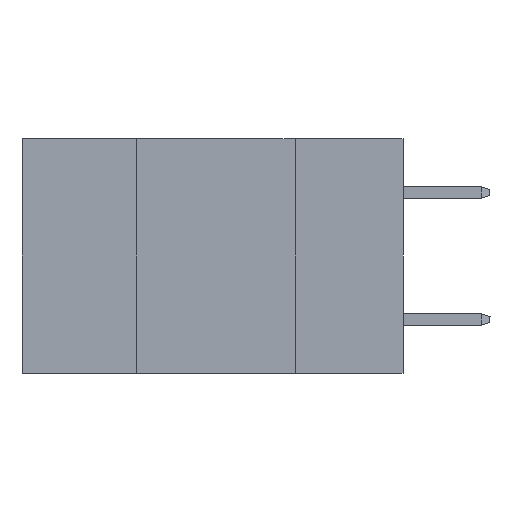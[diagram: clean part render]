
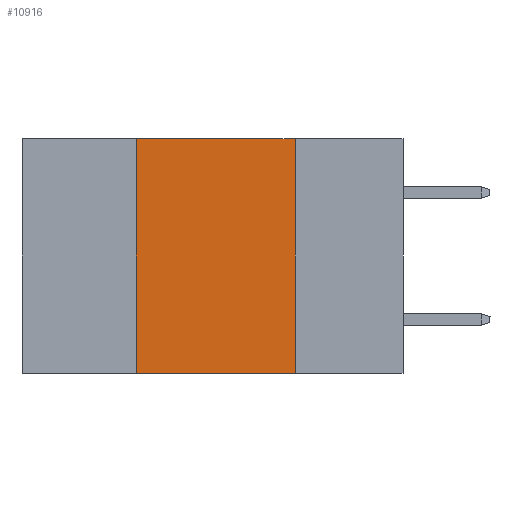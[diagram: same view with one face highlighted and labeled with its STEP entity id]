
A CAD part, left-side view. The second image highlights one B-rep face of the part: STEP entity #10916.
In plain terms, the highlighted planar face has unit normal (-1, 0, 0).
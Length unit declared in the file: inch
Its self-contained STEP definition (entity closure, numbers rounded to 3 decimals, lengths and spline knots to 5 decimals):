
#1675 = DIRECTION ( 'NONE',  ( 1., 0., 0. ) ) ;
#2633 = ORIENTED_EDGE ( 'NONE', *, *, #18885, .F. ) ;
#2917 = VECTOR ( 'NONE', #20141, 39.37008 ) ;
#5406 = LINE ( 'NONE', #11990, #14922 ) ;
#6867 = EDGE_CURVE ( 'NONE', #15799, #18424, #5406, .T. ) ;
#7306 = LINE ( 'NONE', #20338, #10211 ) ;
#7468 = EDGE_LOOP ( 'NONE', ( #17156, #2633, #8340, #9857 ) ) ;
#7472 = VECTOR ( 'NONE', #13784, 39.37008 ) ;
#7933 = FACE_OUTER_BOUND ( 'NONE', #7468, .T. ) ;
#8136 = VERTEX_POINT ( 'NONE', #20972 ) ;
#8340 = ORIENTED_EDGE ( 'NONE', *, *, #14727, .F. ) ;
#8934 = LINE ( 'NONE', #11950, #7472 ) ;
#9857 = ORIENTED_EDGE ( 'NONE', *, *, #11999, .T. ) ;
#9863 = PLANE ( 'NONE',  #14648 ) ;
#10211 = VECTOR ( 'NONE', #13676, 39.37008 ) ;
#10916 = ADVANCED_FACE ( 'NONE', ( #7933 ), #9863, .F. ) ;
#11162 = CARTESIAN_POINT ( 'NONE',  ( 0., 0.6, 0. ) ) ;
#11702 = CARTESIAN_POINT ( 'NONE',  ( 0., 0.17, -0.37 ) ) ;
#11835 = CARTESIAN_POINT ( 'NONE',  ( 0., 0.42, 0. ) ) ;
#11950 = CARTESIAN_POINT ( 'NONE',  ( 0., 0.42, 0. ) ) ;
#11990 = CARTESIAN_POINT ( 'NONE',  ( 0., 0.17, 0. ) ) ;
#11999 = EDGE_CURVE ( 'NONE', #8136, #18424, #7306, .T. ) ;
#13385 = LINE ( 'NONE', #18405, #2917 ) ;
#13676 = DIRECTION ( 'NONE',  ( 0., -1., 0. ) ) ;
#13784 = DIRECTION ( 'NONE',  ( 0., 0., 1. ) ) ;
#14450 = CARTESIAN_POINT ( 'NONE',  ( 0., 0.17, 0. ) ) ;
#14648 = AXIS2_PLACEMENT_3D ( 'NONE', #11162, #1675, #14929 ) ;
#14727 = EDGE_CURVE ( 'NONE', #8136, #19361, #8934, .T. ) ;
#14922 = VECTOR ( 'NONE', #15660, 39.37008 ) ;
#14929 = DIRECTION ( 'NONE',  ( 0., 0., -1. ) ) ;
#15660 = DIRECTION ( 'NONE',  ( 0., 0., -1. ) ) ;
#15799 = VERTEX_POINT ( 'NONE', #14450 ) ;
#17156 = ORIENTED_EDGE ( 'NONE', *, *, #6867, .F. ) ;
#18405 = CARTESIAN_POINT ( 'NONE',  ( 0., 0.6, 0. ) ) ;
#18424 = VERTEX_POINT ( 'NONE', #11702 ) ;
#18885 = EDGE_CURVE ( 'NONE', #19361, #15799, #13385, .T. ) ;
#19361 = VERTEX_POINT ( 'NONE', #11835 ) ;
#20141 = DIRECTION ( 'NONE',  ( 0., -1., 0. ) ) ;
#20338 = CARTESIAN_POINT ( 'NONE',  ( 0., 0.6, -0.37 ) ) ;
#20972 = CARTESIAN_POINT ( 'NONE',  ( 0., 0.42, -0.37 ) ) ;
